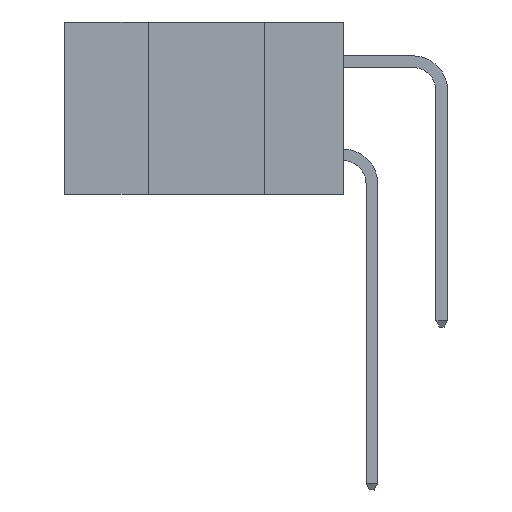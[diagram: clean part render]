
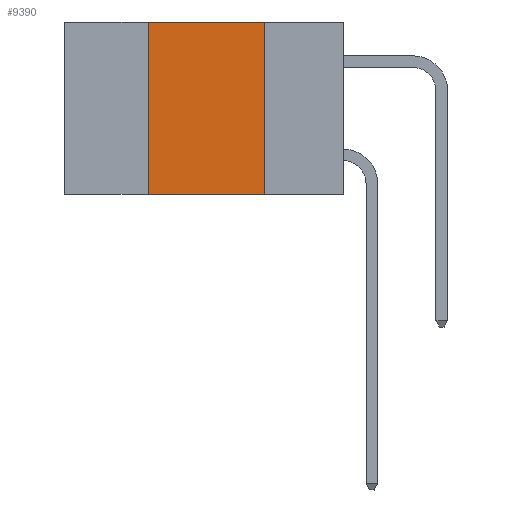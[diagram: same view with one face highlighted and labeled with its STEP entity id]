
A CAD part, left-side view. The second image highlights one B-rep face of the part: STEP entity #9390.
In plain terms, the highlighted planar face has unit normal (-1, 0, 0).
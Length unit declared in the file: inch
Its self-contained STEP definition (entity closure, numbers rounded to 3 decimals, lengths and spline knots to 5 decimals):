
#375 = CARTESIAN_POINT ( 'NONE',  ( 0., 0.6, -0.37 ) ) ;
#784 = CARTESIAN_POINT ( 'NONE',  ( 0., 0.42, -0.37 ) ) ;
#951 = LINE ( 'NONE', #9236, #7001 ) ;
#2443 = LINE ( 'NONE', #12171, #8338 ) ;
#2612 = ORIENTED_EDGE ( 'NONE', *, *, #7629, .F. ) ;
#3258 = DIRECTION ( 'NONE',  ( 0., 0., 1. ) ) ;
#3627 = EDGE_LOOP ( 'NONE', ( #2612, #11469, #6886, #9249 ) ) ;
#3915 = LINE ( 'NONE', #9387, #11875 ) ;
#3931 = LINE ( 'NONE', #375, #7278 ) ;
#4073 = DIRECTION ( 'NONE',  ( 0., 0., -1. ) ) ;
#4389 = VERTEX_POINT ( 'NONE', #5118 ) ;
#5030 = DIRECTION ( 'NONE',  ( 0., 0., -1. ) ) ;
#5118 = CARTESIAN_POINT ( 'NONE',  ( 0., 0.42, 0. ) ) ;
#5124 = VERTEX_POINT ( 'NONE', #12465 ) ;
#5209 = EDGE_CURVE ( 'NONE', #9978, #4389, #3915, .T. ) ;
#6799 = VERTEX_POINT ( 'NONE', #9137 ) ;
#6886 = ORIENTED_EDGE ( 'NONE', *, *, #5209, .F. ) ;
#7001 = VECTOR ( 'NONE', #9412, 39.37008 ) ;
#7278 = VECTOR ( 'NONE', #11424, 39.37008 ) ;
#7629 = EDGE_CURVE ( 'NONE', #5124, #6799, #2443, .T. ) ;
#8059 = CARTESIAN_POINT ( 'NONE',  ( 0., 0.6, 0. ) ) ;
#8338 = VECTOR ( 'NONE', #5030, 39.37008 ) ;
#8799 = FACE_OUTER_BOUND ( 'NONE', #3627, .T. ) ;
#9137 = CARTESIAN_POINT ( 'NONE',  ( 0., 0.17, -0.37 ) ) ;
#9236 = CARTESIAN_POINT ( 'NONE',  ( 0., 0.6, 0. ) ) ;
#9249 = ORIENTED_EDGE ( 'NONE', *, *, #12094, .T. ) ;
#9387 = CARTESIAN_POINT ( 'NONE',  ( 0., 0.42, 0. ) ) ;
#9390 = ADVANCED_FACE ( 'NONE', ( #8799 ), #10264, .F. ) ;
#9412 = DIRECTION ( 'NONE',  ( 0., -1., 0. ) ) ;
#9978 = VERTEX_POINT ( 'NONE', #784 ) ;
#10225 = DIRECTION ( 'NONE',  ( 1., 0., 0. ) ) ;
#10264 = PLANE ( 'NONE',  #12921 ) ;
#10467 = EDGE_CURVE ( 'NONE', #4389, #5124, #951, .T. ) ;
#11424 = DIRECTION ( 'NONE',  ( 0., -1., 0. ) ) ;
#11469 = ORIENTED_EDGE ( 'NONE', *, *, #10467, .F. ) ;
#11875 = VECTOR ( 'NONE', #3258, 39.37008 ) ;
#12094 = EDGE_CURVE ( 'NONE', #9978, #6799, #3931, .T. ) ;
#12171 = CARTESIAN_POINT ( 'NONE',  ( 0., 0.17, 0. ) ) ;
#12465 = CARTESIAN_POINT ( 'NONE',  ( 0., 0.17, 0. ) ) ;
#12921 = AXIS2_PLACEMENT_3D ( 'NONE', #8059, #10225, #4073 ) ;
